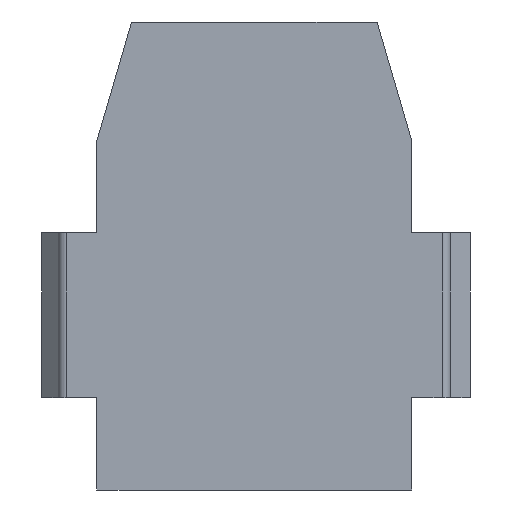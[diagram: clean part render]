
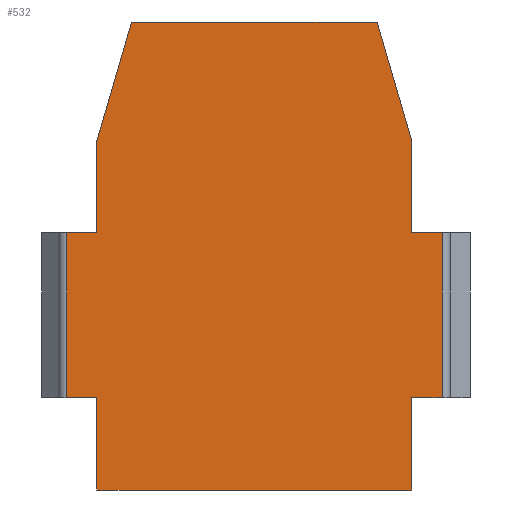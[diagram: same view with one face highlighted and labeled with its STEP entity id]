
A CAD part, front view. The second image highlights one B-rep face of the part: STEP entity #532.
In plain terms, the highlighted planar face has unit normal (0, -1, 0).
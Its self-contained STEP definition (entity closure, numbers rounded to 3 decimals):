
#2 = EDGE_CURVE ( 'NONE', #554, #705, #655, .T. ) ;
#5 = EDGE_CURVE ( 'NONE', #710, #683, #656, .T. ) ;
#12 = EDGE_CURVE ( 'NONE', #673, #590, #871, .T. ) ;
#20 = EDGE_CURVE ( 'NONE', #681, #715, #832, .T. ) ;
#45 = DIRECTION ( 'NONE',  ( 1., 0., 0. ) ) ;
#57 = DIRECTION ( 'NONE',  ( 0.281, 0., 0.96 ) ) ;
#60 = DIRECTION ( 'NONE',  ( 0., 0., -1. ) ) ;
#61 = CARTESIAN_POINT ( 'NONE',  ( -10.975, 0., -4.95 ) ) ;
#66 = DIRECTION ( 'NONE',  ( 0., 0., 1. ) ) ;
#67 = DIRECTION ( 'NONE',  ( -1., 0., 0. ) ) ;
#78 = DIRECTION ( 'NONE',  ( 1., 0., 0. ) ) ;
#79 = CARTESIAN_POINT ( 'NONE',  ( -10.975, 0., 4.95 ) ) ;
#85 = CARTESIAN_POINT ( 'NONE',  ( -7.375, 0., 17.6 ) ) ;
#86 = CARTESIAN_POINT ( 'NONE',  ( 11.275, 0., 4.95 ) ) ;
#89 = CARTESIAN_POINT ( 'NONE',  ( -7.375, 0., 17.6 ) ) ;
#93 = DIRECTION ( 'NONE',  ( 0., 0., 1. ) ) ;
#97 = CARTESIAN_POINT ( 'NONE',  ( -9.45, 0., 4.95 ) ) ;
#100 = DIRECTION ( 'NONE',  ( 1., 0., 0. ) ) ;
#120 = CARTESIAN_POINT ( 'NONE',  ( 9.45, 0., 4.95 ) ) ;
#128 = CARTESIAN_POINT ( 'NONE',  ( 9.45, 0., -4.95 ) ) ;
#133 = CARTESIAN_POINT ( 'NONE',  ( -11.275, 0., -4.95 ) ) ;
#143 = DIRECTION ( 'NONE',  ( -1., 0., 0. ) ) ;
#144 = CARTESIAN_POINT ( 'NONE',  ( -9.45, 0., -10.5 ) ) ;
#145 = DIRECTION ( 'NONE',  ( 0., 0., 1. ) ) ;
#168 = AXIS2_PLACEMENT_3D ( 'NONE', #354, #340, #339 ) ;
#226 = EDGE_CURVE ( 'NONE', #705, #676, #835, .T. ) ;
#230 = EDGE_CURVE ( 'NONE', #715, #668, #1005, .T. ) ;
#239 = EDGE_CURVE ( 'NONE', #710, #590, #910, .T. ) ;
#240 = EDGE_CURVE ( 'NONE', #679, #676, #898, .T. ) ;
#241 = EDGE_CURVE ( 'NONE', #668, #670, #1014, .T. ) ;
#248 = EDGE_CURVE ( 'NONE', #679, #681, #908, .T. ) ;
#270 = CARTESIAN_POINT ( 'NONE',  ( -9.45, 0., 10.5 ) ) ;
#275 = CARTESIAN_POINT ( 'NONE',  ( 11.275, 0., -4.95 ) ) ;
#278 = DIRECTION ( 'NONE',  ( 0., 0., -1. ) ) ;
#281 = CARTESIAN_POINT ( 'NONE',  ( 9.45, 0., 4.95 ) ) ;
#282 = CARTESIAN_POINT ( 'NONE',  ( -9.45, 0., -4.95 ) ) ;
#299 = CARTESIAN_POINT ( 'NONE',  ( 9.45, 0., -10.5 ) ) ;
#307 = CARTESIAN_POINT ( 'NONE',  ( 9.45, 0., -4.95 ) ) ;
#309 = CARTESIAN_POINT ( 'NONE',  ( -9.45, 0., 4.95 ) ) ;
#312 = CARTESIAN_POINT ( 'NONE',  ( -11.275, 0., 4.95 ) ) ;
#315 = DIRECTION ( 'NONE',  ( 0.281, 0., -0.96 ) ) ;
#317 = CARTESIAN_POINT ( 'NONE',  ( -11.275, 0., -4.95 ) ) ;
#321 = CARTESIAN_POINT ( 'NONE',  ( 9.45, 0., 10.5 ) ) ;
#323 = CARTESIAN_POINT ( 'NONE',  ( 7.375, 0., 17.6 ) ) ;
#324 = CARTESIAN_POINT ( 'NONE',  ( -7.375, 0., 17.6 ) ) ;
#327 = CARTESIAN_POINT ( 'NONE',  ( 7.375, 0., 17.6 ) ) ;
#334 = CARTESIAN_POINT ( 'NONE',  ( -9.45, 0., -10.5 ) ) ;
#337 = CARTESIAN_POINT ( 'NONE',  ( 9.45, 0., 4.95 ) ) ;
#339 = DIRECTION ( 'NONE',  ( 0., 0., -1. ) ) ;
#340 = DIRECTION ( 'NONE',  ( 0., -1., 0. ) ) ;
#342 = CARTESIAN_POINT ( 'NONE',  ( 11.275, 0., 4.95 ) ) ;
#343 = PLANE ( 'NONE',  #168 ) ;
#350 = DIRECTION ( 'NONE',  ( 0., 0., -1. ) ) ;
#351 = CARTESIAN_POINT ( 'NONE',  ( 9.45, 0., -10.5 ) ) ;
#354 = CARTESIAN_POINT ( 'NONE',  ( 0., 0., 0. ) ) ;
#480 = DIRECTION ( 'NONE',  ( -1., 0., 0. ) ) ;
#481 = CARTESIAN_POINT ( 'NONE',  ( -9.45, 0., -10.5 ) ) ;
#489 = EDGE_CURVE ( 'NONE', #670, #674, #947, .T. ) ;
#493 = EDGE_CURVE ( 'NONE', #674, #673, #935, .T. ) ;
#496 = EDGE_CURVE ( 'NONE', #683, #689, #931, .T. ) ;
#500 = EDGE_CURVE ( 'NONE', #689, #554, #914, .T. ) ;
#532 = ADVANCED_FACE ( 'NONE', ( #842 ), #343, .T. ) ;
#554 = VERTEX_POINT ( 'NONE', #334 ) ;
#590 = VERTEX_POINT ( 'NONE', #342 ) ;
#646 = VECTOR ( 'NONE', #143, 1000. ) ;
#649 = EDGE_LOOP ( 'NONE', ( #714, #717, #718, #719, #720, #721, #722, #723, #724, #793, #768, #764, #727, #767 ) ) ;
#654 = VECTOR ( 'NONE', #145, 1000. ) ;
#655 = LINE ( 'NONE', #144, #654 ) ;
#656 = LINE ( 'NONE', #128, #646 ) ;
#668 = VERTEX_POINT ( 'NONE', #324 ) ;
#670 = VERTEX_POINT ( 'NONE', #323 ) ;
#673 = VERTEX_POINT ( 'NONE', #337 ) ;
#674 = VERTEX_POINT ( 'NONE', #321 ) ;
#676 = VERTEX_POINT ( 'NONE', #317 ) ;
#679 = VERTEX_POINT ( 'NONE', #312 ) ;
#681 = VERTEX_POINT ( 'NONE', #309 ) ;
#683 = VERTEX_POINT ( 'NONE', #307 ) ;
#689 = VERTEX_POINT ( 'NONE', #299 ) ;
#705 = VERTEX_POINT ( 'NONE', #282 ) ;
#710 = VERTEX_POINT ( 'NONE', #275 ) ;
#714 = ORIENTED_EDGE ( 'NONE', *, *, #5, .F. ) ;
#715 = VERTEX_POINT ( 'NONE', #270 ) ;
#717 = ORIENTED_EDGE ( 'NONE', *, *, #239, .T. ) ;
#718 = ORIENTED_EDGE ( 'NONE', *, *, #12, .F. ) ;
#719 = ORIENTED_EDGE ( 'NONE', *, *, #493, .F. ) ;
#720 = ORIENTED_EDGE ( 'NONE', *, *, #489, .F. ) ;
#721 = ORIENTED_EDGE ( 'NONE', *, *, #241, .F. ) ;
#722 = ORIENTED_EDGE ( 'NONE', *, *, #230, .F. ) ;
#723 = ORIENTED_EDGE ( 'NONE', *, *, #20, .F. ) ;
#724 = ORIENTED_EDGE ( 'NONE', *, *, #248, .F. ) ;
#727 = ORIENTED_EDGE ( 'NONE', *, *, #500, .F. ) ;
#764 = ORIENTED_EDGE ( 'NONE', *, *, #2, .F. ) ;
#767 = ORIENTED_EDGE ( 'NONE', *, *, #496, .F. ) ;
#768 = ORIENTED_EDGE ( 'NONE', *, *, #226, .F. ) ;
#793 = ORIENTED_EDGE ( 'NONE', *, *, #240, .T. ) ;
#832 = LINE ( 'NONE', #97, #840 ) ;
#835 = LINE ( 'NONE', #61, #1000 ) ;
#840 = VECTOR ( 'NONE', #93, 1000. ) ;
#842 = FACE_OUTER_BOUND ( 'NONE', #649, .T. ) ;
#869 = VECTOR ( 'NONE', #45, 1000. ) ;
#871 = LINE ( 'NONE', #120, #869 ) ;
#898 = LINE ( 'NONE', #133, #996 ) ;
#905 = VECTOR ( 'NONE', #66, 1000. ) ;
#908 = LINE ( 'NONE', #79, #976 ) ;
#910 = LINE ( 'NONE', #86, #905 ) ;
#914 = LINE ( 'NONE', #481, #921 ) ;
#921 = VECTOR ( 'NONE', #480, 1000. ) ;
#928 = VECTOR ( 'NONE', #350, 1000. ) ;
#931 = LINE ( 'NONE', #351, #928 ) ;
#935 = LINE ( 'NONE', #281, #938 ) ;
#938 = VECTOR ( 'NONE', #278, 1000. ) ;
#940 = VECTOR ( 'NONE', #315, 1000. ) ;
#947 = LINE ( 'NONE', #327, #940 ) ;
#976 = VECTOR ( 'NONE', #78, 1000. ) ;
#994 = VECTOR ( 'NONE', #100, 1000. ) ;
#996 = VECTOR ( 'NONE', #60, 1000. ) ;
#1000 = VECTOR ( 'NONE', #67, 1000. ) ;
#1005 = LINE ( 'NONE', #89, #1009 ) ;
#1009 = VECTOR ( 'NONE', #57, 1000. ) ;
#1014 = LINE ( 'NONE', #85, #994 ) ;
